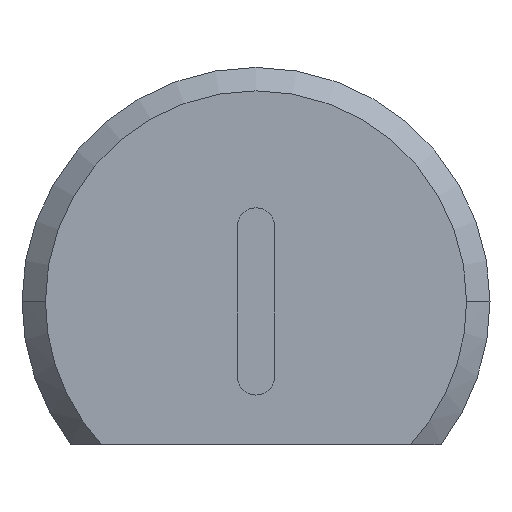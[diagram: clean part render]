
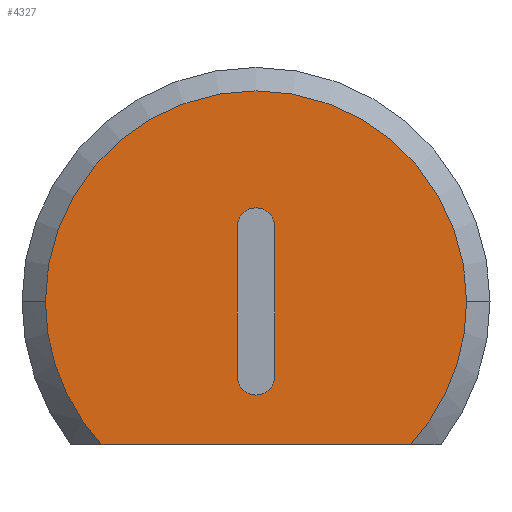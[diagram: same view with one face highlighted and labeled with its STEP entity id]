
A CAD part, front view. The second image highlights one B-rep face of the part: STEP entity #4327.
In plain terms, the highlighted planar face has unit normal (0, -1, 0).
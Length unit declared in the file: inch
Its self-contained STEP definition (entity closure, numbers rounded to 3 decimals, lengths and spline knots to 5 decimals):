
#30 = DIRECTION ( 'NONE',  ( -1., 0., 0. ) ) ;
#153 = CARTESIAN_POINT ( 'NONE',  ( 0.02, -0.075, -0.08 ) ) ;
#321 = EDGE_CURVE ( 'NONE', #4582, #4481, #2579, .T. ) ;
#341 = LINE ( 'NONE', #4482, #4883 ) ;
#387 = ORIENTED_EDGE ( 'NONE', *, *, #1835, .T. ) ;
#440 = DIRECTION ( 'NONE',  ( 0., -1., 0. ) ) ;
#478 = CARTESIAN_POINT ( 'NONE',  ( -0.225, -0.075, 0. ) ) ;
#555 = AXIS2_PLACEMENT_3D ( 'NONE', #852, #2947, #30 ) ;
#588 = CARTESIAN_POINT ( 'NONE',  ( -0.02, -0.075, 0.08 ) ) ;
#591 = EDGE_CURVE ( 'NONE', #4067, #5220, #1276, .T. ) ;
#852 = CARTESIAN_POINT ( 'NONE',  ( 0., -0.075, 0.08 ) ) ;
#1124 = FACE_BOUND ( 'NONE', #2522, .T. ) ;
#1224 = CARTESIAN_POINT ( 'NONE',  ( 0.225, -0.075, 0. ) ) ;
#1276 = CIRCLE ( 'NONE', #5193, 0.02 ) ;
#1287 = DIRECTION ( 'NONE',  ( 0., -1., 0. ) ) ;
#1309 = DIRECTION ( 'NONE',  ( 0., 0., -1. ) ) ;
#1312 = AXIS2_PLACEMENT_3D ( 'NONE', #3337, #2976, #2107 ) ;
#1410 = VERTEX_POINT ( 'NONE', #588 ) ;
#1422 = ORIENTED_EDGE ( 'NONE', *, *, #5104, .F. ) ;
#1533 = VERTEX_POINT ( 'NONE', #4505 ) ;
#1598 = ORIENTED_EDGE ( 'NONE', *, *, #3751, .T. ) ;
#1612 = EDGE_CURVE ( 'NONE', #1673, #1410, #2674, .T. ) ;
#1628 = LINE ( 'NONE', #3715, #2467 ) ;
#1673 = VERTEX_POINT ( 'NONE', #4226 ) ;
#1762 = DIRECTION ( 'NONE',  ( 0., -1., 0. ) ) ;
#1813 = CIRCLE ( 'NONE', #4207, 0.225 ) ;
#1835 = EDGE_CURVE ( 'NONE', #3303, #1533, #1813, .T. ) ;
#2081 = DIRECTION ( 'NONE',  ( -1., 0., 0. ) ) ;
#2090 = DIRECTION ( 'NONE',  ( 0., -1., 0. ) ) ;
#2107 = DIRECTION ( 'NONE',  ( -1., 0., 0. ) ) ;
#2111 = CARTESIAN_POINT ( 'NONE',  ( 0., -0.075, 0. ) ) ;
#2248 = ORIENTED_EDGE ( 'NONE', *, *, #2517, .F. ) ;
#2467 = VECTOR ( 'NONE', #4132, 39.37008 ) ;
#2517 = EDGE_CURVE ( 'NONE', #5220, #1673, #341, .T. ) ;
#2522 = EDGE_LOOP ( 'NONE', ( #4467, #2248, #4456, #3378 ) ) ;
#2579 = CIRCLE ( 'NONE', #1312, 0.225 ) ;
#2613 = CARTESIAN_POINT ( 'NONE',  ( 0., -0.075, -0.08 ) ) ;
#2674 = CIRCLE ( 'NONE', #555, 0.02 ) ;
#2773 = EDGE_LOOP ( 'NONE', ( #1422, #5314, #1598, #387 ) ) ;
#2947 = DIRECTION ( 'NONE',  ( 0., -1., 0. ) ) ;
#2976 = DIRECTION ( 'NONE',  ( 0., -1., 0. ) ) ;
#3131 = AXIS2_PLACEMENT_3D ( 'NONE', #2111, #440, #2081 ) ;
#3303 = VERTEX_POINT ( 'NONE', #478 ) ;
#3337 = CARTESIAN_POINT ( 'NONE',  ( 0., -0.075, 0. ) ) ;
#3378 = ORIENTED_EDGE ( 'NONE', *, *, #4089, .F. ) ;
#3381 = PLANE ( 'NONE',  #3488 ) ;
#3477 = CARTESIAN_POINT ( 'NONE',  ( 0., -0.075, 0. ) ) ;
#3488 = AXIS2_PLACEMENT_3D ( 'NONE', #3827, #2090, #3780 ) ;
#3625 = CARTESIAN_POINT ( 'NONE',  ( 0.16507, -0.075, -0.1529 ) ) ;
#3678 = LINE ( 'NONE', #4527, #4299 ) ;
#3715 = CARTESIAN_POINT ( 'NONE',  ( -0.19779, -0.075, -0.1529 ) ) ;
#3751 = EDGE_CURVE ( 'NONE', #4481, #3303, #4119, .T. ) ;
#3780 = DIRECTION ( 'NONE',  ( -1., 0., 0. ) ) ;
#3827 = CARTESIAN_POINT ( 'NONE',  ( 0., -0.075, 0. ) ) ;
#4067 = VERTEX_POINT ( 'NONE', #5352 ) ;
#4089 = EDGE_CURVE ( 'NONE', #1410, #4067, #3678, .T. ) ;
#4093 = DIRECTION ( 'NONE',  ( 0., 0., 1. ) ) ;
#4119 = CIRCLE ( 'NONE', #3131, 0.225 ) ;
#4132 = DIRECTION ( 'NONE',  ( -1., 0., 0. ) ) ;
#4195 = DIRECTION ( 'NONE',  ( -1., 0., 0. ) ) ;
#4207 = AXIS2_PLACEMENT_3D ( 'NONE', #3477, #1762, #4652 ) ;
#4226 = CARTESIAN_POINT ( 'NONE',  ( 0.02, -0.075, 0.08 ) ) ;
#4299 = VECTOR ( 'NONE', #1309, 39.37008 ) ;
#4327 = ADVANCED_FACE ( 'NONE', ( #5332, #1124 ), #3381, .T. ) ;
#4456 = ORIENTED_EDGE ( 'NONE', *, *, #591, .F. ) ;
#4467 = ORIENTED_EDGE ( 'NONE', *, *, #1612, .F. ) ;
#4481 = VERTEX_POINT ( 'NONE', #1224 ) ;
#4482 = CARTESIAN_POINT ( 'NONE',  ( 0.02, -0.075, 0.08 ) ) ;
#4505 = CARTESIAN_POINT ( 'NONE',  ( -0.16507, -0.075, -0.1529 ) ) ;
#4527 = CARTESIAN_POINT ( 'NONE',  ( -0.02, -0.075, 0.08 ) ) ;
#4582 = VERTEX_POINT ( 'NONE', #3625 ) ;
#4652 = DIRECTION ( 'NONE',  ( -1., 0., 0. ) ) ;
#4883 = VECTOR ( 'NONE', #4093, 39.37008 ) ;
#5104 = EDGE_CURVE ( 'NONE', #4582, #1533, #1628, .T. ) ;
#5193 = AXIS2_PLACEMENT_3D ( 'NONE', #2613, #1287, #4195 ) ;
#5220 = VERTEX_POINT ( 'NONE', #153 ) ;
#5314 = ORIENTED_EDGE ( 'NONE', *, *, #321, .T. ) ;
#5332 = FACE_OUTER_BOUND ( 'NONE', #2773, .T. ) ;
#5352 = CARTESIAN_POINT ( 'NONE',  ( -0.02, -0.075, -0.08 ) ) ;
